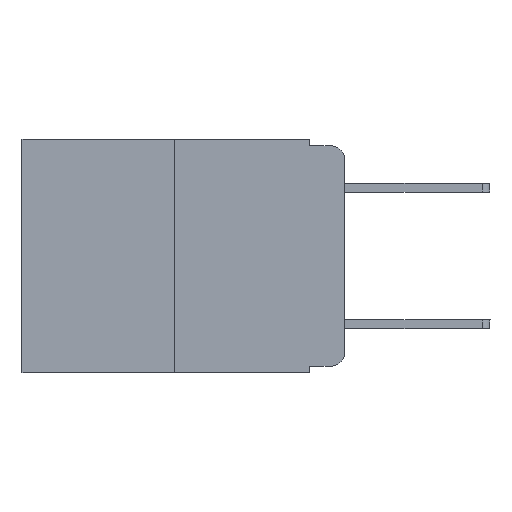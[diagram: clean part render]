
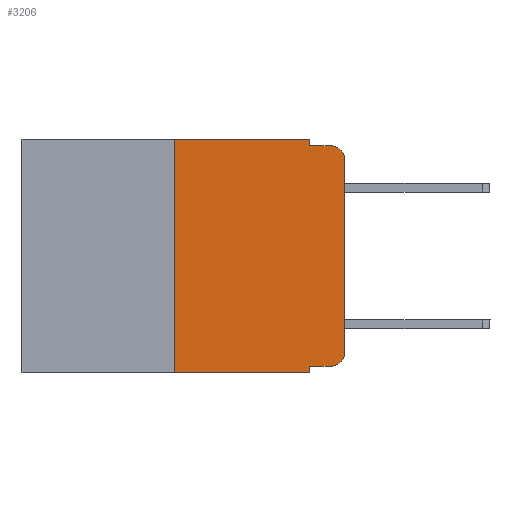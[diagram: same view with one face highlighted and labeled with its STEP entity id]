
A CAD part, left-side view. The second image highlights one B-rep face of the part: STEP entity #3206.
In plain terms, the highlighted planar face has unit normal (-1, 0, 0).
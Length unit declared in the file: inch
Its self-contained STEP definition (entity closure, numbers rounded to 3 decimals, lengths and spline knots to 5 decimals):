
#35 = VERTEX_POINT ( 'NONE', #2456 ) ;
#457 = CARTESIAN_POINT ( 'NONE',  ( 0., 0.473, 0. ) ) ;
#460 = EDGE_CURVE ( 'NONE', #5593, #8128, #9658, .T. ) ;
#538 = EDGE_CURVE ( 'NONE', #8440, #5593, #1039, .T. ) ;
#633 = CARTESIAN_POINT ( 'NONE',  ( 0., 0.051, -0.01 ) ) ;
#1030 = CARTESIAN_POINT ( 'NONE',  ( 0., 0.25, 0. ) ) ;
#1039 = LINE ( 'NONE', #8003, #12209 ) ;
#1122 = DIRECTION ( 'NONE',  ( 0., 0., 1. ) ) ;
#1137 = VECTOR ( 'NONE', #3718, 39.37008 ) ;
#1429 = CARTESIAN_POINT ( 'NONE',  ( 0., 0.051, 0. ) ) ;
#1539 = VERTEX_POINT ( 'NONE', #10844 ) ;
#1675 = EDGE_CURVE ( 'NONE', #8891, #8128, #10465, .T. ) ;
#1895 = ORIENTED_EDGE ( 'NONE', *, *, #1675, .T. ) ;
#1948 = DIRECTION ( 'NONE',  ( -1., 0., 0. ) ) ;
#2084 = VECTOR ( 'NONE', #7230, 39.37008 ) ;
#2216 = CARTESIAN_POINT ( 'NONE',  ( 0., 0.02, -0.03 ) ) ;
#2260 = DIRECTION ( 'NONE',  ( 0., 0., -1. ) ) ;
#2297 = EDGE_CURVE ( 'NONE', #2838, #35, #6406, .T. ) ;
#2338 = AXIS2_PLACEMENT_3D ( 'NONE', #5484, #13038, #2260 ) ;
#2456 = CARTESIAN_POINT ( 'NONE',  ( 0., 0.051, -0.343 ) ) ;
#2647 = EDGE_CURVE ( 'NONE', #2838, #5744, #12480, .T. ) ;
#2651 = LINE ( 'NONE', #4964, #13632 ) ;
#2838 = VERTEX_POINT ( 'NONE', #8168 ) ;
#2841 = EDGE_CURVE ( 'NONE', #4417, #8440, #10932, .T. ) ;
#3206 = ADVANCED_FACE ( 'NONE', ( #9901 ), #9334, .F. ) ;
#3563 = CARTESIAN_POINT ( 'NONE',  ( 0., 0.25, 0. ) ) ;
#3718 = DIRECTION ( 'NONE',  ( 0., -1., 0. ) ) ;
#4054 = ORIENTED_EDGE ( 'NONE', *, *, #2647, .T. ) ;
#4417 = VERTEX_POINT ( 'NONE', #3563 ) ;
#4634 = EDGE_CURVE ( 'NONE', #5744, #5286, #9918, .T. ) ;
#4964 = CARTESIAN_POINT ( 'NONE',  ( 0., 0.473, -0.343 ) ) ;
#5019 = EDGE_CURVE ( 'NONE', #1539, #35, #2651, .T. ) ;
#5145 = AXIS2_PLACEMENT_3D ( 'NONE', #2216, #6576, #7646 ) ;
#5264 = DIRECTION ( 'NONE',  ( 0., 0., -1. ) ) ;
#5286 = VERTEX_POINT ( 'NONE', #8558 ) ;
#5484 = CARTESIAN_POINT ( 'NONE',  ( 0., 0.473, 0. ) ) ;
#5592 = ORIENTED_EDGE ( 'NONE', *, *, #460, .F. ) ;
#5593 = VERTEX_POINT ( 'NONE', #12258 ) ;
#5744 = VERTEX_POINT ( 'NONE', #6858 ) ;
#6073 = DIRECTION ( 'NONE',  ( 0., -1., 0. ) ) ;
#6347 = AXIS2_PLACEMENT_3D ( 'NONE', #7337, #1948, #5264 ) ;
#6406 = LINE ( 'NONE', #9618, #11476 ) ;
#6442 = EDGE_LOOP ( 'NONE', ( #7392, #1895, #5592, #10877, #9325, #7384, #12565, #8399, #4054, #8682 ) ) ;
#6576 = DIRECTION ( 'NONE',  ( -1., 0., 0. ) ) ;
#6710 = EDGE_CURVE ( 'NONE', #5286, #8891, #10015, .T. ) ;
#6801 = VECTOR ( 'NONE', #8046, 39.37008 ) ;
#6858 = CARTESIAN_POINT ( 'NONE',  ( 0., 0.02, -0.333 ) ) ;
#7230 = DIRECTION ( 'NONE',  ( 0., 0., 1. ) ) ;
#7337 = CARTESIAN_POINT ( 'NONE',  ( 0., 0.02, -0.313 ) ) ;
#7384 = ORIENTED_EDGE ( 'NONE', *, *, #7561, .F. ) ;
#7392 = ORIENTED_EDGE ( 'NONE', *, *, #6710, .T. ) ;
#7561 = EDGE_CURVE ( 'NONE', #1539, #4417, #7977, .T. ) ;
#7646 = DIRECTION ( 'NONE',  ( 0., 0., -1. ) ) ;
#7691 = CARTESIAN_POINT ( 'NONE',  ( 0., 0., -0.03 ) ) ;
#7977 = LINE ( 'NONE', #1030, #9506 ) ;
#8003 = CARTESIAN_POINT ( 'NONE',  ( 0., 0.051, 0. ) ) ;
#8046 = DIRECTION ( 'NONE',  ( 0., -1., 0. ) ) ;
#8128 = VERTEX_POINT ( 'NONE', #9434 ) ;
#8168 = CARTESIAN_POINT ( 'NONE',  ( 0., 0.051, -0.333 ) ) ;
#8399 = ORIENTED_EDGE ( 'NONE', *, *, #2297, .F. ) ;
#8440 = VERTEX_POINT ( 'NONE', #1429 ) ;
#8558 = CARTESIAN_POINT ( 'NONE',  ( 0., 0., -0.313 ) ) ;
#8682 = ORIENTED_EDGE ( 'NONE', *, *, #4634, .T. ) ;
#8749 = CARTESIAN_POINT ( 'NONE',  ( 0., 0.051, -0.333 ) ) ;
#8891 = VERTEX_POINT ( 'NONE', #7691 ) ;
#9325 = ORIENTED_EDGE ( 'NONE', *, *, #2841, .F. ) ;
#9334 = PLANE ( 'NONE',  #2338 ) ;
#9434 = CARTESIAN_POINT ( 'NONE',  ( 0., 0.02, -0.01 ) ) ;
#9506 = VECTOR ( 'NONE', #1122, 39.37008 ) ;
#9618 = CARTESIAN_POINT ( 'NONE',  ( 0., 0.051, 0. ) ) ;
#9658 = LINE ( 'NONE', #633, #6801 ) ;
#9901 = FACE_OUTER_BOUND ( 'NONE', #6442, .T. ) ;
#9908 = DIRECTION ( 'NONE',  ( 0., -1., 0. ) ) ;
#9918 = CIRCLE ( 'NONE', #6347, 0.02 ) ;
#10015 = LINE ( 'NONE', #10353, #2084 ) ;
#10182 = DIRECTION ( 'NONE',  ( 0., 0., -1. ) ) ;
#10353 = CARTESIAN_POINT ( 'NONE',  ( 0., 0., 0. ) ) ;
#10465 = CIRCLE ( 'NONE', #5145, 0.02 ) ;
#10713 = DIRECTION ( 'NONE',  ( 0., 0., -1. ) ) ;
#10844 = CARTESIAN_POINT ( 'NONE',  ( 0., 0.25, -0.343 ) ) ;
#10877 = ORIENTED_EDGE ( 'NONE', *, *, #538, .F. ) ;
#10932 = LINE ( 'NONE', #457, #1137 ) ;
#11476 = VECTOR ( 'NONE', #10713, 39.37008 ) ;
#12209 = VECTOR ( 'NONE', #10182, 39.37008 ) ;
#12258 = CARTESIAN_POINT ( 'NONE',  ( 0., 0.051, -0.01 ) ) ;
#12480 = LINE ( 'NONE', #8749, #13142 ) ;
#12565 = ORIENTED_EDGE ( 'NONE', *, *, #5019, .T. ) ;
#13038 = DIRECTION ( 'NONE',  ( 1., 0., 0. ) ) ;
#13142 = VECTOR ( 'NONE', #9908, 39.37008 ) ;
#13632 = VECTOR ( 'NONE', #6073, 39.37008 ) ;
